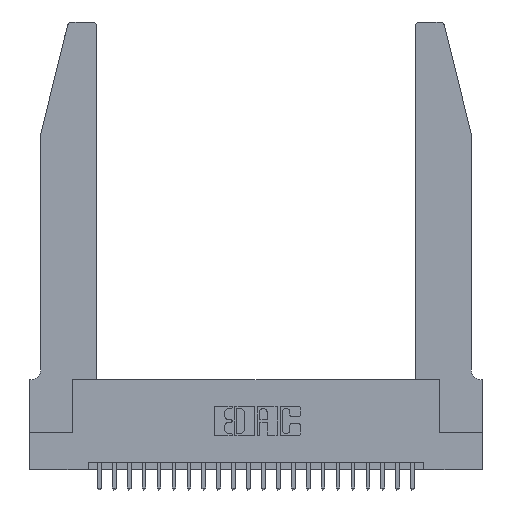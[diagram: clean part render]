
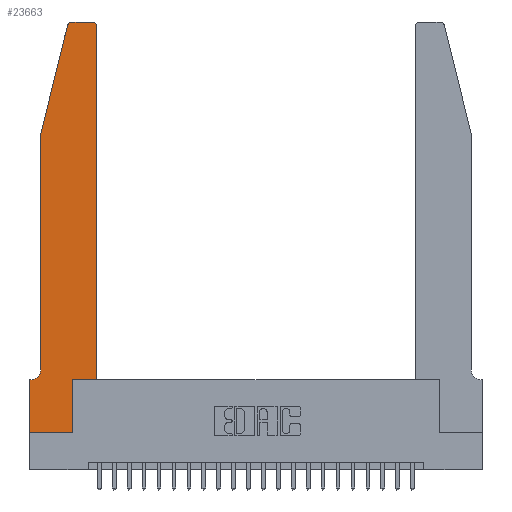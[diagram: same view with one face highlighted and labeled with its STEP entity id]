
A CAD part, top view. The second image highlights one B-rep face of the part: STEP entity #23663.
In plain terms, the highlighted planar face has unit normal (0, 0, 1).
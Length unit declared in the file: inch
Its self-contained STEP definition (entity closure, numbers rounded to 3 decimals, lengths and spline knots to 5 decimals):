
#163 = DIRECTION ( 'NONE',  ( 0., 0., 1. ) ) ;
#251 = ORIENTED_EDGE ( 'NONE', *, *, #21936, .T. ) ;
#368 = CARTESIAN_POINT ( 'NONE',  ( 0.0055, 0.42, 0.37 ) ) ;
#530 = VECTOR ( 'NONE', #1749, 39.37008 ) ;
#842 = AXIS2_PLACEMENT_3D ( 'NONE', #11728, #163, #13587 ) ;
#1178 = DIRECTION ( 'NONE',  ( 0., -1., 0. ) ) ;
#1217 = CARTESIAN_POINT ( 'NONE',  ( 0.0755, 2., 0.37 ) ) ;
#1222 = CARTESIAN_POINT ( 'NONE',  ( 0.4505, 2.72, 0.37 ) ) ;
#1302 = LINE ( 'NONE', #19670, #20961 ) ;
#1653 = DIRECTION ( 'NONE',  ( -1., 0., 0. ) ) ;
#1749 = DIRECTION ( 'NONE',  ( 0., 1., 0. ) ) ;
#1791 = VERTEX_POINT ( 'NONE', #24260 ) ;
#2338 = EDGE_CURVE ( 'NONE', #23797, #17375, #21351, .T. ) ;
#2346 = DIRECTION ( 'NONE',  ( -1., 0., 0. ) ) ;
#2557 = VECTOR ( 'NONE', #12408, 39.37008 ) ;
#3306 = CARTESIAN_POINT ( 'NONE',  ( 0.0055, 0.35, 0.37 ) ) ;
#3446 = EDGE_CURVE ( 'NONE', #17678, #5623, #13899, .T. ) ;
#3662 = ORIENTED_EDGE ( 'NONE', *, *, #4804, .T. ) ;
#4042 = EDGE_CURVE ( 'NONE', #15852, #20564, #1302, .T. ) ;
#4132 = EDGE_CURVE ( 'NONE', #9404, #24326, #24247, .T. ) ;
#4442 = CARTESIAN_POINT ( 'NONE',  ( 0.0755, 2., 0.37 ) ) ;
#4611 = DIRECTION ( 'NONE',  ( 1., 0., 0. ) ) ;
#4721 = CARTESIAN_POINT ( 'NONE',  ( 0., 0., 0.37 ) ) ;
#4804 = EDGE_CURVE ( 'NONE', #16093, #17678, #15922, .T. ) ;
#4856 = CARTESIAN_POINT ( 'NONE',  ( 0.4205, 2.72, 0.37 ) ) ;
#5623 = VERTEX_POINT ( 'NONE', #14982 ) ;
#5641 = VECTOR ( 'NONE', #12388, 39.37008 ) ;
#5673 = AXIS2_PLACEMENT_3D ( 'NONE', #368, #13773, #2346 ) ;
#5872 = VECTOR ( 'NONE', #16010, 39.37008 ) ;
#6291 = CARTESIAN_POINT ( 'NONE',  ( 0.4505, 0.35, 0.37 ) ) ;
#6428 = VERTEX_POINT ( 'NONE', #18869 ) ;
#6658 = CARTESIAN_POINT ( 'NONE',  ( 0.0755, 0.42, 0.37 ) ) ;
#6796 = DIRECTION ( 'NONE',  ( 1., 0., 0. ) ) ;
#6841 = VECTOR ( 'NONE', #1178, 39.37008 ) ;
#6867 = ORIENTED_EDGE ( 'NONE', *, *, #4132, .T. ) ;
#7683 = VERTEX_POINT ( 'NONE', #3306 ) ;
#8424 = ORIENTED_EDGE ( 'NONE', *, *, #20292, .T. ) ;
#8645 = CIRCLE ( 'NONE', #5673, 0.07 ) ;
#9017 = VECTOR ( 'NONE', #18534, 39.37008 ) ;
#9394 = CARTESIAN_POINT ( 'NONE',  ( 0.284, 2.72, 0.37 ) ) ;
#9404 = VERTEX_POINT ( 'NONE', #1222 ) ;
#9433 = CARTESIAN_POINT ( 'NONE',  ( 0., 0.35, 0.37 ) ) ;
#10403 = LINE ( 'NONE', #13112, #14760 ) ;
#10450 = CARTESIAN_POINT ( 'NONE',  ( 0., 0., 0.37 ) ) ;
#10856 = EDGE_CURVE ( 'NONE', #6428, #23797, #17524, .T. ) ;
#10866 = EDGE_CURVE ( 'NONE', #20564, #9404, #11375, .T. ) ;
#11307 = DIRECTION ( 'NONE',  ( 1., 0., 0. ) ) ;
#11375 = LINE ( 'NONE', #20713, #530 ) ;
#11542 = ORIENTED_EDGE ( 'NONE', *, *, #15020, .T. ) ;
#11728 = CARTESIAN_POINT ( 'NONE',  ( 0., 0.35, 0.37 ) ) ;
#12388 = DIRECTION ( 'NONE',  ( 0., 1., 0. ) ) ;
#12408 = DIRECTION ( 'NONE',  ( 1., 0., 0. ) ) ;
#12776 = ORIENTED_EDGE ( 'NONE', *, *, #3446, .T. ) ;
#13112 = CARTESIAN_POINT ( 'NONE',  ( 0.0755, 0.35, 0.37 ) ) ;
#13587 = DIRECTION ( 'NONE',  ( 1., 0., 0. ) ) ;
#13773 = DIRECTION ( 'NONE',  ( 0., 0., -1. ) ) ;
#13899 = LINE ( 'NONE', #4721, #2557 ) ;
#14018 = ORIENTED_EDGE ( 'NONE', *, *, #2338, .T. ) ;
#14150 = EDGE_CURVE ( 'NONE', #17375, #7683, #8645, .T. ) ;
#14280 = EDGE_CURVE ( 'NONE', #5623, #15852, #17466, .T. ) ;
#14760 = VECTOR ( 'NONE', #1653, 39.37008 ) ;
#14982 = CARTESIAN_POINT ( 'NONE',  ( 0.2865, 0., 0.37 ) ) ;
#15020 = EDGE_CURVE ( 'NONE', #7683, #16093, #10403, .T. ) ;
#15078 = EDGE_LOOP ( 'NONE', ( #251, #8424, #18720, #14018, #22998, #11542, #3662, #12776, #23375, #23415, #21821, #6867 ) ) ;
#15852 = VERTEX_POINT ( 'NONE', #21892 ) ;
#15922 = LINE ( 'NONE', #10450, #5872 ) ;
#16010 = DIRECTION ( 'NONE',  ( 0., -1., 0. ) ) ;
#16025 = FACE_OUTER_BOUND ( 'NONE', #15078, .T. ) ;
#16093 = VERTEX_POINT ( 'NONE', #9433 ) ;
#16872 = DIRECTION ( 'NONE',  ( -0.239, -0.971, 0. ) ) ;
#17375 = VERTEX_POINT ( 'NONE', #6658 ) ;
#17466 = LINE ( 'NONE', #23710, #5641 ) ;
#17524 = LINE ( 'NONE', #22511, #20803 ) ;
#17678 = VERTEX_POINT ( 'NONE', #21118 ) ;
#18071 = DIRECTION ( 'NONE',  ( 0., 0., 1. ) ) ;
#18457 = AXIS2_PLACEMENT_3D ( 'NONE', #9394, #22572, #11307 ) ;
#18534 = DIRECTION ( 'NONE',  ( -1., 0., 0. ) ) ;
#18720 = ORIENTED_EDGE ( 'NONE', *, *, #10856, .T. ) ;
#18869 = CARTESIAN_POINT ( 'NONE',  ( 0.25487, 2.72718, 0.37 ) ) ;
#19003 = LINE ( 'NONE', #24338, #9017 ) ;
#19670 = CARTESIAN_POINT ( 'NONE',  ( 0.4505, 0.35, 0.37 ) ) ;
#20292 = EDGE_CURVE ( 'NONE', #1791, #6428, #24513, .T. ) ;
#20564 = VERTEX_POINT ( 'NONE', #6291 ) ;
#20713 = CARTESIAN_POINT ( 'NONE',  ( 0.4505, 0.35, 0.37 ) ) ;
#20803 = VECTOR ( 'NONE', #16872, 39.37008 ) ;
#20961 = VECTOR ( 'NONE', #4611, 39.37008 ) ;
#21118 = CARTESIAN_POINT ( 'NONE',  ( 0., 0., 0.37 ) ) ;
#21351 = LINE ( 'NONE', #1217, #6841 ) ;
#21821 = ORIENTED_EDGE ( 'NONE', *, *, #10866, .T. ) ;
#21892 = CARTESIAN_POINT ( 'NONE',  ( 0.2865, 0.35, 0.37 ) ) ;
#21936 = EDGE_CURVE ( 'NONE', #24326, #1791, #19003, .T. ) ;
#22511 = CARTESIAN_POINT ( 'NONE',  ( 0.0755, 2., 0.37 ) ) ;
#22572 = DIRECTION ( 'NONE',  ( 0., 0., 1. ) ) ;
#22925 = PLANE ( 'NONE',  #842 ) ;
#22998 = ORIENTED_EDGE ( 'NONE', *, *, #14150, .T. ) ;
#23375 = ORIENTED_EDGE ( 'NONE', *, *, #14280, .T. ) ;
#23415 = ORIENTED_EDGE ( 'NONE', *, *, #4042, .T. ) ;
#23493 = CARTESIAN_POINT ( 'NONE',  ( 0.4205, 2.75, 0.37 ) ) ;
#23663 = ADVANCED_FACE ( 'NONE', ( #16025 ), #22925, .T. ) ;
#23710 = CARTESIAN_POINT ( 'NONE',  ( 0.2865, 0.35, 0.37 ) ) ;
#23797 = VERTEX_POINT ( 'NONE', #4442 ) ;
#24247 = CIRCLE ( 'NONE', #24607, 0.03 ) ;
#24260 = CARTESIAN_POINT ( 'NONE',  ( 0.284, 2.75, 0.37 ) ) ;
#24326 = VERTEX_POINT ( 'NONE', #23493 ) ;
#24338 = CARTESIAN_POINT ( 'NONE',  ( 0.2605, 2.75, 0.37 ) ) ;
#24513 = CIRCLE ( 'NONE', #18457, 0.03 ) ;
#24607 = AXIS2_PLACEMENT_3D ( 'NONE', #4856, #18071, #6796 ) ;
